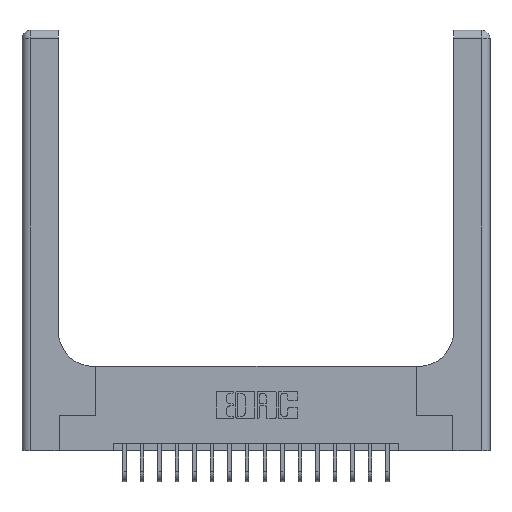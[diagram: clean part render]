
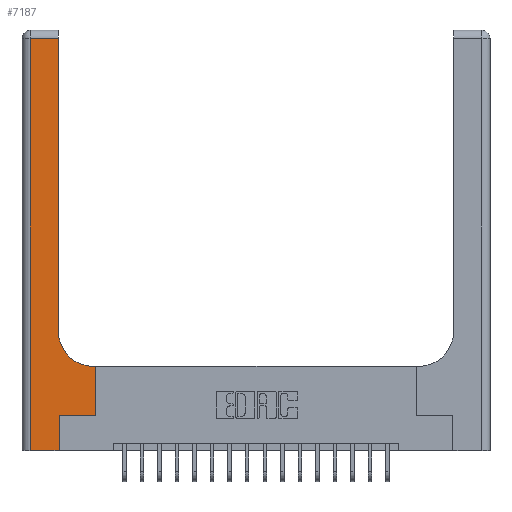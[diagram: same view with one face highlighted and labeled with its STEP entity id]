
A CAD part, top view. The second image highlights one B-rep face of the part: STEP entity #7187.
In plain terms, the highlighted planar face has unit normal (0, 0, 1).
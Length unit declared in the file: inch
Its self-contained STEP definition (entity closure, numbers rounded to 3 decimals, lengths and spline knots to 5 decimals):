
#257 = CARTESIAN_POINT ( 'NONE',  ( 0., 0., 0.37 ) ) ;
#378 = DIRECTION ( 'NONE',  ( 0., 1., 0. ) ) ;
#990 = VECTOR ( 'NONE', #13581, 39.37008 ) ;
#1346 = EDGE_CURVE ( 'NONE', #16215, #17692, #18547, .T. ) ;
#1379 = CIRCLE ( 'NONE', #1785, 0.25 ) ;
#1785 = AXIS2_PLACEMENT_3D ( 'NONE', #7810, #14298, #11048 ) ;
#1918 = DIRECTION ( 'NONE',  ( 1., 0., 0. ) ) ;
#1990 = LINE ( 'NONE', #2003, #11804 ) ;
#2003 = CARTESIAN_POINT ( 'NONE',  ( 0.26, 3., 0.37 ) ) ;
#2260 = CARTESIAN_POINT ( 'NONE',  ( 0.26, 2.94, 0.37 ) ) ;
#3340 = LINE ( 'NONE', #257, #8894 ) ;
#3381 = AXIS2_PLACEMENT_3D ( 'NONE', #14753, #11353, #19664 ) ;
#3602 = CARTESIAN_POINT ( 'NONE',  ( 0.26, 0.85, 0.37 ) ) ;
#4846 = CARTESIAN_POINT ( 'NONE',  ( 0.528, 0.6, 0.37 ) ) ;
#5596 = EDGE_LOOP ( 'NONE', ( #20260, #16067, #15096, #17571, #19342, #18981, #16223, #11637, #5982 ) ) ;
#5625 = DIRECTION ( 'NONE',  ( 0., 1., 0. ) ) ;
#5841 = CARTESIAN_POINT ( 'NONE',  ( 0.265, 0.25, 0.37 ) ) ;
#5982 = ORIENTED_EDGE ( 'NONE', *, *, #18581, .T. ) ;
#6585 = EDGE_CURVE ( 'NONE', #17692, #11026, #18113, .T. ) ;
#6624 = VECTOR ( 'NONE', #8061, 39.37008 ) ;
#6641 = DIRECTION ( 'NONE',  ( 1., 0., 0. ) ) ;
#7099 = CARTESIAN_POINT ( 'NONE',  ( 0.528, 0.25, 0.37 ) ) ;
#7108 = VERTEX_POINT ( 'NONE', #19107 ) ;
#7187 = ADVANCED_FACE ( 'NONE', ( #18876 ), #9797, .F. ) ;
#7314 = VECTOR ( 'NONE', #1918, 39.37008 ) ;
#7810 = CARTESIAN_POINT ( 'NONE',  ( 0.51, 0.85, 0.37 ) ) ;
#8061 = DIRECTION ( 'NONE',  ( -1., 0., 0. ) ) ;
#8734 = VERTEX_POINT ( 'NONE', #5841 ) ;
#8894 = VECTOR ( 'NONE', #6641, 39.37008 ) ;
#9087 = EDGE_CURVE ( 'NONE', #11026, #20315, #3340, .T. ) ;
#9797 = PLANE ( 'NONE',  #3381 ) ;
#10430 = CARTESIAN_POINT ( 'NONE',  ( 0.265, 0., 0.37 ) ) ;
#10548 = CARTESIAN_POINT ( 'NONE',  ( 0.528, 0.25, 0.37 ) ) ;
#10772 = CARTESIAN_POINT ( 'NONE',  ( 0.265, 0., 0.37 ) ) ;
#11026 = VERTEX_POINT ( 'NONE', #18516 ) ;
#11048 = DIRECTION ( 'NONE',  ( 1., 0., 0. ) ) ;
#11353 = DIRECTION ( 'NONE',  ( 0., 0., -1. ) ) ;
#11637 = ORIENTED_EDGE ( 'NONE', *, *, #15043, .T. ) ;
#11804 = VECTOR ( 'NONE', #378, 39.37008 ) ;
#11840 = LINE ( 'NONE', #11922, #19736 ) ;
#11922 = CARTESIAN_POINT ( 'NONE',  ( 0.26, 0.6, 0.37 ) ) ;
#11970 = EDGE_CURVE ( 'NONE', #19575, #17115, #14363, .T. ) ;
#12890 = VECTOR ( 'NONE', #5625, 39.37008 ) ;
#13113 = VERTEX_POINT ( 'NONE', #3602 ) ;
#13581 = DIRECTION ( 'NONE',  ( 0., 1., 0. ) ) ;
#13623 = EDGE_CURVE ( 'NONE', #8734, #19575, #18710, .T. ) ;
#13833 = EDGE_CURVE ( 'NONE', #20315, #8734, #13876, .T. ) ;
#13876 = LINE ( 'NONE', #10430, #12890 ) ;
#14298 = DIRECTION ( 'NONE',  ( 0., 0., -1. ) ) ;
#14363 = LINE ( 'NONE', #10548, #990 ) ;
#14753 = CARTESIAN_POINT ( 'NONE',  ( 0., 3., 0.37 ) ) ;
#15043 = EDGE_CURVE ( 'NONE', #17115, #7108, #11840, .T. ) ;
#15055 = CARTESIAN_POINT ( 'NONE',  ( 0.06, 3., 0.37 ) ) ;
#15096 = ORIENTED_EDGE ( 'NONE', *, *, #6585, .T. ) ;
#15601 = EDGE_CURVE ( 'NONE', #13113, #16215, #1990, .T. ) ;
#16067 = ORIENTED_EDGE ( 'NONE', *, *, #1346, .T. ) ;
#16203 = CARTESIAN_POINT ( 'NONE',  ( 0.06, 2.94, 0.37 ) ) ;
#16215 = VERTEX_POINT ( 'NONE', #2260 ) ;
#16223 = ORIENTED_EDGE ( 'NONE', *, *, #11970, .T. ) ;
#16328 = CARTESIAN_POINT ( 'NONE',  ( 0., 2.94, 0.37 ) ) ;
#16588 = VECTOR ( 'NONE', #18448, 39.37008 ) ;
#16889 = DIRECTION ( 'NONE',  ( -1., 0., 0. ) ) ;
#17115 = VERTEX_POINT ( 'NONE', #4846 ) ;
#17571 = ORIENTED_EDGE ( 'NONE', *, *, #9087, .T. ) ;
#17692 = VERTEX_POINT ( 'NONE', #16203 ) ;
#18113 = LINE ( 'NONE', #15055, #16588 ) ;
#18448 = DIRECTION ( 'NONE',  ( 0., -1., 0. ) ) ;
#18516 = CARTESIAN_POINT ( 'NONE',  ( 0.06, 0., 0.37 ) ) ;
#18547 = LINE ( 'NONE', #16328, #6624 ) ;
#18581 = EDGE_CURVE ( 'NONE', #7108, #13113, #1379, .T. ) ;
#18710 = LINE ( 'NONE', #19474, #7314 ) ;
#18876 = FACE_OUTER_BOUND ( 'NONE', #5596, .T. ) ;
#18981 = ORIENTED_EDGE ( 'NONE', *, *, #13623, .T. ) ;
#19107 = CARTESIAN_POINT ( 'NONE',  ( 0.51, 0.6, 0.37 ) ) ;
#19342 = ORIENTED_EDGE ( 'NONE', *, *, #13833, .T. ) ;
#19474 = CARTESIAN_POINT ( 'NONE',  ( 0.265, 0.25, 0.37 ) ) ;
#19575 = VERTEX_POINT ( 'NONE', #7099 ) ;
#19664 = DIRECTION ( 'NONE',  ( -1., 0., 0. ) ) ;
#19736 = VECTOR ( 'NONE', #16889, 39.37008 ) ;
#20260 = ORIENTED_EDGE ( 'NONE', *, *, #15601, .T. ) ;
#20315 = VERTEX_POINT ( 'NONE', #10772 ) ;
